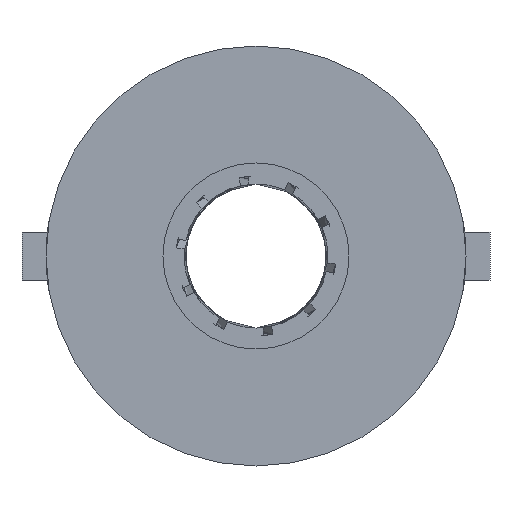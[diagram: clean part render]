
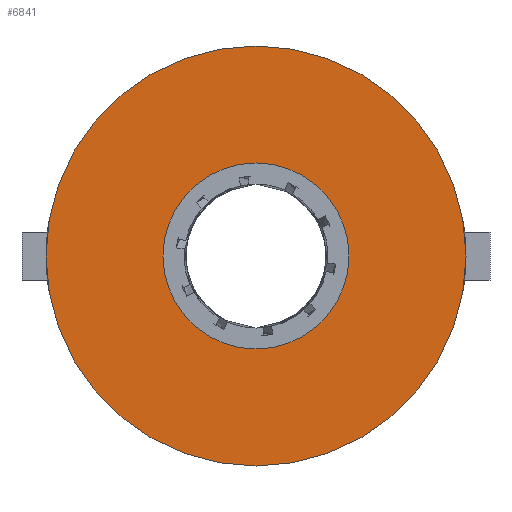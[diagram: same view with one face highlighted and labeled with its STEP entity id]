
A CAD part, front view. The second image highlights one B-rep face of the part: STEP entity #6841.
In plain terms, the highlighted planar face has unit normal (0, -1, 0).
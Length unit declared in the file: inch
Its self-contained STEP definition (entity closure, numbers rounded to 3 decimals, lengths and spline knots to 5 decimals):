
#197 = CARTESIAN_POINT ( 'NONE',  ( 0., 0., 0. ) ) ;
#676 = ORIENTED_EDGE ( 'NONE', *, *, #4899, .T. ) ;
#689 = FACE_OUTER_BOUND ( 'NONE', #9229, .T. ) ;
#917 = ORIENTED_EDGE ( 'NONE', *, *, #3114, .T. ) ;
#1414 = AXIS2_PLACEMENT_3D ( 'NONE', #7224, #3391, #8724 ) ;
#1443 = CARTESIAN_POINT ( 'NONE',  ( 0., 0., -0.155 ) ) ;
#1814 = AXIS2_PLACEMENT_3D ( 'NONE', #197, #5458, #6138 ) ;
#2314 = AXIS2_PLACEMENT_3D ( 'NONE', #3049, #9071, #7691 ) ;
#2490 = CARTESIAN_POINT ( 'NONE',  ( 0., 0., 0. ) ) ;
#3049 = CARTESIAN_POINT ( 'NONE',  ( 0., 0., 0. ) ) ;
#3114 = EDGE_CURVE ( 'NONE', #8661, #8519, #6486, .T. ) ;
#3179 = AXIS2_PLACEMENT_3D ( 'NONE', #2490, #9202, #5455 ) ;
#3391 = DIRECTION ( 'NONE',  ( 0., 1., 0. ) ) ;
#3486 = VERTEX_POINT ( 'NONE', #6796 ) ;
#4427 = DIRECTION ( 'NONE',  ( 0., 1., 0. ) ) ;
#4651 = CIRCLE ( 'NONE', #3179, 0.35 ) ;
#4826 = CARTESIAN_POINT ( 'NONE',  ( 0., 0., 0.35 ) ) ;
#4899 = EDGE_CURVE ( 'NONE', #3486, #7281, #4651, .T. ) ;
#5217 = PLANE ( 'NONE',  #7974 ) ;
#5252 = DIRECTION ( 'NONE',  ( 0., 0., 1. ) ) ;
#5455 = DIRECTION ( 'NONE',  ( 0., 0., -1. ) ) ;
#5456 = CARTESIAN_POINT ( 'NONE',  ( 0., 0., 0.155 ) ) ;
#5458 = DIRECTION ( 'NONE',  ( 0., 1., 0. ) ) ;
#5853 = FACE_BOUND ( 'NONE', #6478, .T. ) ;
#6138 = DIRECTION ( 'NONE',  ( 0., 0., 1. ) ) ;
#6177 = ORIENTED_EDGE ( 'NONE', *, *, #7650, .T. ) ;
#6478 = EDGE_LOOP ( 'NONE', ( #6177, #917 ) ) ;
#6486 = CIRCLE ( 'NONE', #1414, 0.155 ) ;
#6796 = CARTESIAN_POINT ( 'NONE',  ( 0., 0., -0.35 ) ) ;
#6841 = ADVANCED_FACE ( 'NONE', ( #5853, #689 ), #5217, .F. ) ;
#7224 = CARTESIAN_POINT ( 'NONE',  ( 0., 0., 0. ) ) ;
#7281 = VERTEX_POINT ( 'NONE', #4826 ) ;
#7650 = EDGE_CURVE ( 'NONE', #8519, #8661, #7965, .T. ) ;
#7691 = DIRECTION ( 'NONE',  ( 0., 0., -1. ) ) ;
#7833 = EDGE_CURVE ( 'NONE', #7281, #3486, #9603, .T. ) ;
#7965 = CIRCLE ( 'NONE', #1814, 0.155 ) ;
#7974 = AXIS2_PLACEMENT_3D ( 'NONE', #8938, #4427, #5252 ) ;
#8430 = ORIENTED_EDGE ( 'NONE', *, *, #7833, .T. ) ;
#8519 = VERTEX_POINT ( 'NONE', #1443 ) ;
#8661 = VERTEX_POINT ( 'NONE', #5456 ) ;
#8724 = DIRECTION ( 'NONE',  ( 0., 0., 1. ) ) ;
#8938 = CARTESIAN_POINT ( 'NONE',  ( 0., 0., 0. ) ) ;
#9071 = DIRECTION ( 'NONE',  ( 0., -1., 0. ) ) ;
#9202 = DIRECTION ( 'NONE',  ( 0., -1., 0. ) ) ;
#9229 = EDGE_LOOP ( 'NONE', ( #676, #8430 ) ) ;
#9603 = CIRCLE ( 'NONE', #2314, 0.35 ) ;
